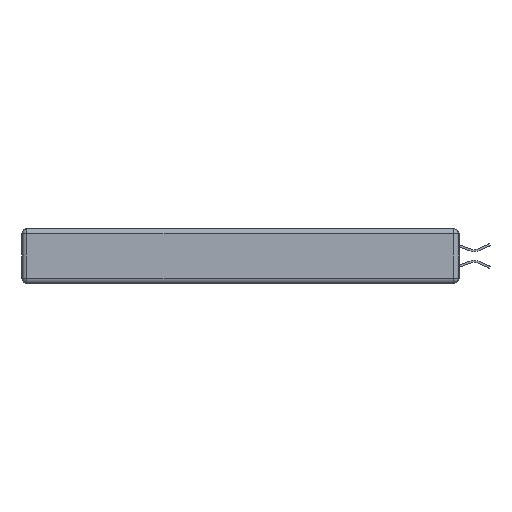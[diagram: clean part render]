
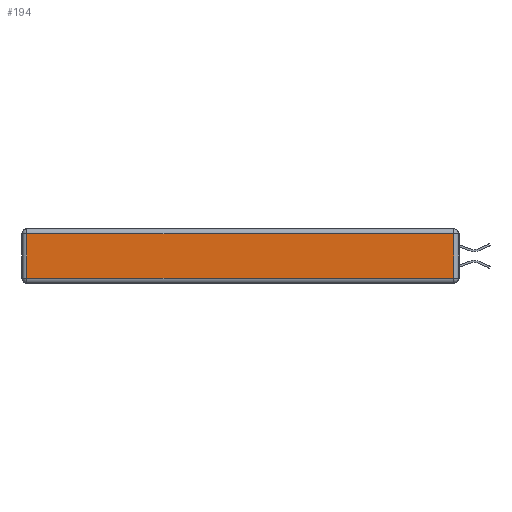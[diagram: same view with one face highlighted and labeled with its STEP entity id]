
A CAD part, left-side view. The second image highlights one B-rep face of the part: STEP entity #194.
In plain terms, the highlighted planar face has unit normal (-1, 0, 0).
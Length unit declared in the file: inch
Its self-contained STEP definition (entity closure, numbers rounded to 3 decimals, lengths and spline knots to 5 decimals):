
#176 = VECTOR ( 'NONE', #2207, 39.37008 ) ;
#194 = ADVANCED_FACE ( 'NONE', ( #17775 ), #24525, .T. ) ;
#207 = LINE ( 'NONE', #15313, #5735 ) ;
#565 = CARTESIAN_POINT ( 'NONE',  ( 0., 2.72, -0.03 ) ) ;
#871 = CARTESIAN_POINT ( 'NONE',  ( 0., 2.72, -0.313 ) ) ;
#2207 = DIRECTION ( 'NONE',  ( 0., 0., 1. ) ) ;
#3088 = CARTESIAN_POINT ( 'NONE',  ( 0., 0., -0.343 ) ) ;
#3369 = ORIENTED_EDGE ( 'NONE', *, *, #4157, .T. ) ;
#3400 = ORIENTED_EDGE ( 'NONE', *, *, #7515, .T. ) ;
#4157 = EDGE_CURVE ( 'NONE', #17957, #9413, #11009, .T. ) ;
#4358 = DIRECTION ( 'NONE',  ( 0., 1., 0. ) ) ;
#5735 = VECTOR ( 'NONE', #9543, 39.37008 ) ;
#6008 = EDGE_LOOP ( 'NONE', ( #3400, #12984, #19711, #3369 ) ) ;
#7053 = DIRECTION ( 'NONE',  ( 0., 0., 1. ) ) ;
#7128 = CARTESIAN_POINT ( 'NONE',  ( 0., 0.03, -0.313 ) ) ;
#7324 = VECTOR ( 'NONE', #20100, 39.37008 ) ;
#7515 = EDGE_CURVE ( 'NONE', #9413, #15287, #207, .T. ) ;
#9413 = VERTEX_POINT ( 'NONE', #871 ) ;
#9421 = LINE ( 'NONE', #9887, #176 ) ;
#9543 = DIRECTION ( 'NONE',  ( 0., -1., 0. ) ) ;
#9887 = CARTESIAN_POINT ( 'NONE',  ( 0., 0.03, -0.343 ) ) ;
#11009 = LINE ( 'NONE', #22152, #7324 ) ;
#12078 = CARTESIAN_POINT ( 'NONE',  ( 0., 2.75, -0.03 ) ) ;
#12984 = ORIENTED_EDGE ( 'NONE', *, *, #13568, .T. ) ;
#13568 = EDGE_CURVE ( 'NONE', #15287, #15357, #9421, .T. ) ;
#15041 = LINE ( 'NONE', #12078, #20925 ) ;
#15287 = VERTEX_POINT ( 'NONE', #7128 ) ;
#15313 = CARTESIAN_POINT ( 'NONE',  ( 0., 0., -0.313 ) ) ;
#15357 = VERTEX_POINT ( 'NONE', #21203 ) ;
#17739 = AXIS2_PLACEMENT_3D ( 'NONE', #3088, #18792, #7053 ) ;
#17775 = FACE_OUTER_BOUND ( 'NONE', #6008, .T. ) ;
#17933 = EDGE_CURVE ( 'NONE', #15357, #17957, #15041, .T. ) ;
#17957 = VERTEX_POINT ( 'NONE', #565 ) ;
#18792 = DIRECTION ( 'NONE',  ( -1., 0., 0. ) ) ;
#19711 = ORIENTED_EDGE ( 'NONE', *, *, #17933, .T. ) ;
#20100 = DIRECTION ( 'NONE',  ( 0., 0., -1. ) ) ;
#20925 = VECTOR ( 'NONE', #4358, 39.37008 ) ;
#21203 = CARTESIAN_POINT ( 'NONE',  ( 0., 0.03, -0.03 ) ) ;
#22152 = CARTESIAN_POINT ( 'NONE',  ( 0., 2.72, -0.343 ) ) ;
#24525 = PLANE ( 'NONE',  #17739 ) ;
